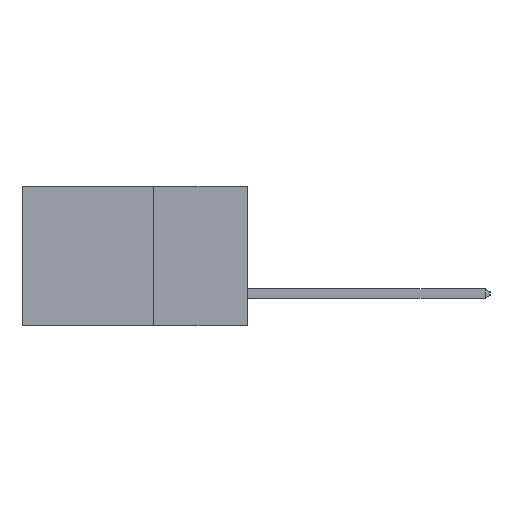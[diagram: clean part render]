
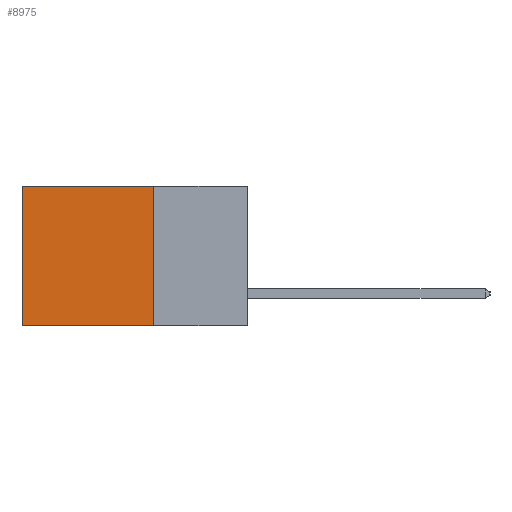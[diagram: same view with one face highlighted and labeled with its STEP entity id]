
A CAD part, left-side view. The second image highlights one B-rep face of the part: STEP entity #8975.
In plain terms, the highlighted planar face has unit normal (-1, 0, 0).
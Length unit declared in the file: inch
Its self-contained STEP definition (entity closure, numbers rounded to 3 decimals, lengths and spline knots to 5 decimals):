
#675 = VECTOR ( 'NONE', #5206, 39.37008 ) ;
#1029 = VECTOR ( 'NONE', #1246, 39.37008 ) ;
#1190 = PLANE ( 'NONE',  #11375 ) ;
#1246 = DIRECTION ( 'NONE',  ( 0., 0., -1. ) ) ;
#1938 = ORIENTED_EDGE ( 'NONE', *, *, #4499, .T. ) ;
#2689 = VECTOR ( 'NONE', #5694, 39.37008 ) ;
#2858 = EDGE_LOOP ( 'NONE', ( #1938, #11199, #11746, #3049 ) ) ;
#3049 = ORIENTED_EDGE ( 'NONE', *, *, #8009, .T. ) ;
#3068 = VERTEX_POINT ( 'NONE', #9342 ) ;
#3502 = CARTESIAN_POINT ( 'NONE',  ( 0.2615, 0.25, -0.37 ) ) ;
#4158 = CARTESIAN_POINT ( 'NONE',  ( 0.2615, 0.6, -0.37 ) ) ;
#4499 = EDGE_CURVE ( 'NONE', #10954, #5658, #11800, .T. ) ;
#5050 = CARTESIAN_POINT ( 'NONE',  ( 0.2615, 0.6, 0. ) ) ;
#5206 = DIRECTION ( 'NONE',  ( 0., 1., 0. ) ) ;
#5463 = LINE ( 'NONE', #8529, #675 ) ;
#5658 = VERTEX_POINT ( 'NONE', #6211 ) ;
#5694 = DIRECTION ( 'NONE',  ( 0., 1., 0. ) ) ;
#6173 = LINE ( 'NONE', #3502, #1029 ) ;
#6211 = CARTESIAN_POINT ( 'NONE',  ( 0.2615, 0.6, -0.37 ) ) ;
#6295 = LINE ( 'NONE', #6683, #2689 ) ;
#6314 = CARTESIAN_POINT ( 'NONE',  ( 0.2615, 0.25, 0. ) ) ;
#6683 = CARTESIAN_POINT ( 'NONE',  ( 0.2615, 0.25, -0.37 ) ) ;
#7543 = EDGE_CURVE ( 'NONE', #11244, #3068, #6173, .T. ) ;
#8009 = EDGE_CURVE ( 'NONE', #11244, #10954, #5463, .T. ) ;
#8529 = CARTESIAN_POINT ( 'NONE',  ( 0.2615, 0.25, 0. ) ) ;
#8863 = CARTESIAN_POINT ( 'NONE',  ( 0.2615, 0.25, -0.37 ) ) ;
#8946 = VECTOR ( 'NONE', #11772, 39.37008 ) ;
#8975 = ADVANCED_FACE ( 'NONE', ( #11450 ), #1190, .F. ) ;
#9342 = CARTESIAN_POINT ( 'NONE',  ( 0.2615, 0.25, -0.37 ) ) ;
#10954 = VERTEX_POINT ( 'NONE', #5050 ) ;
#11199 = ORIENTED_EDGE ( 'NONE', *, *, #11662, .F. ) ;
#11244 = VERTEX_POINT ( 'NONE', #6314 ) ;
#11274 = DIRECTION ( 'NONE',  ( 1., 0., 0. ) ) ;
#11375 = AXIS2_PLACEMENT_3D ( 'NONE', #8863, #11274, #13459 ) ;
#11450 = FACE_OUTER_BOUND ( 'NONE', #2858, .T. ) ;
#11662 = EDGE_CURVE ( 'NONE', #3068, #5658, #6295, .T. ) ;
#11746 = ORIENTED_EDGE ( 'NONE', *, *, #7543, .F. ) ;
#11772 = DIRECTION ( 'NONE',  ( 0., 0., -1. ) ) ;
#11800 = LINE ( 'NONE', #4158, #8946 ) ;
#13459 = DIRECTION ( 'NONE',  ( 0., 0., -1. ) ) ;
